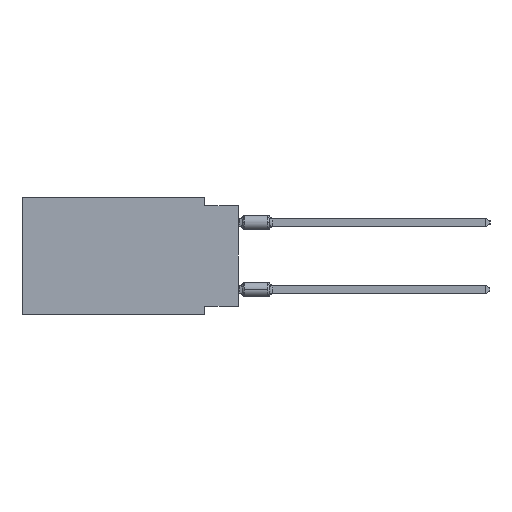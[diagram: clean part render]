
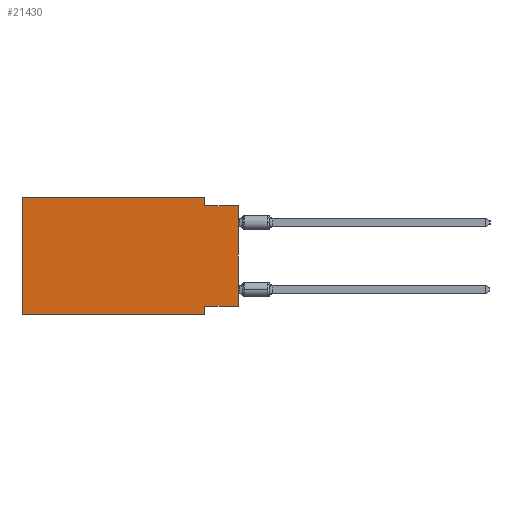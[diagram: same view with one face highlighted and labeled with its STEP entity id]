
A CAD part, left-side view. The second image highlights one B-rep face of the part: STEP entity #21430.
In plain terms, the highlighted planar face has unit normal (-1, 0, 0).
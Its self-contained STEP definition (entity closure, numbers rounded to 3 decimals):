
#437 = PLANE ( 'NONE',  #22385 ) ;
#1089 = LINE ( 'NONE', #18104, #20816 ) ;
#2187 = CARTESIAN_POINT ( 'NONE',  ( 0., 16.383, -8.89 ) ) ;
#2880 = VECTOR ( 'NONE', #39582, 1000. ) ;
#2970 = ORIENTED_EDGE ( 'NONE', *, *, #8130, .T. ) ;
#3034 = EDGE_CURVE ( 'NONE', #49198, #54674, #1089, .T. ) ;
#3231 = VECTOR ( 'NONE', #26576, 1000. ) ;
#4536 = EDGE_CURVE ( 'NONE', #9688, #14217, #16787, .T. ) ;
#5107 = EDGE_CURVE ( 'NONE', #48577, #19049, #5271, .T. ) ;
#5271 = LINE ( 'NONE', #25919, #48688 ) ;
#5369 = ORIENTED_EDGE ( 'NONE', *, *, #5107, .F. ) ;
#6031 = CARTESIAN_POINT ( 'NONE',  ( 0., 0., -0.635 ) ) ;
#6118 = DIRECTION ( 'NONE',  ( 0., 0., 1. ) ) ;
#7225 = CARTESIAN_POINT ( 'NONE',  ( 0., 2.54, -0.635 ) ) ;
#7441 = CARTESIAN_POINT ( 'NONE',  ( 0., 16.383, -8.89 ) ) ;
#8130 = EDGE_CURVE ( 'NONE', #13922, #54674, #41264, .T. ) ;
#9395 = CARTESIAN_POINT ( 'NONE',  ( 0., 2.54, 0. ) ) ;
#9688 = VERTEX_POINT ( 'NONE', #10948 ) ;
#10948 = CARTESIAN_POINT ( 'NONE',  ( 0., 16.383, 0. ) ) ;
#11138 = EDGE_CURVE ( 'NONE', #46643, #49198, #14525, .T. ) ;
#12032 = DIRECTION ( 'NONE',  ( 0., -1., 0. ) ) ;
#13807 = CARTESIAN_POINT ( 'NONE',  ( 0., 2.54, -8.255 ) ) ;
#13908 = EDGE_CURVE ( 'NONE', #13922, #9688, #31509, .T. ) ;
#13922 = VERTEX_POINT ( 'NONE', #2187 ) ;
#14217 = VERTEX_POINT ( 'NONE', #9395 ) ;
#14525 = LINE ( 'NONE', #52854, #3231 ) ;
#16787 = LINE ( 'NONE', #45863, #19187 ) ;
#18097 = ORIENTED_EDGE ( 'NONE', *, *, #24493, .F. ) ;
#18104 = CARTESIAN_POINT ( 'NONE',  ( 0., 2.54, -8.89 ) ) ;
#18314 = LINE ( 'NONE', #35376, #2880 ) ;
#19049 = VERTEX_POINT ( 'NONE', #6031 ) ;
#19088 = VECTOR ( 'NONE', #6118, 1000. ) ;
#19187 = VECTOR ( 'NONE', #12032, 1000. ) ;
#20816 = VECTOR ( 'NONE', #32611, 1000. ) ;
#21430 = ADVANCED_FACE ( 'NONE', ( #38712 ), #437, .F. ) ;
#21928 = CARTESIAN_POINT ( 'NONE',  ( 0., 16.383, 0. ) ) ;
#22385 = AXIS2_PLACEMENT_3D ( 'NONE', #21928, #22477, #51871 ) ;
#22477 = DIRECTION ( 'NONE',  ( 1., 0., 0. ) ) ;
#24463 = DIRECTION ( 'NONE',  ( 0., -1., 0. ) ) ;
#24493 = EDGE_CURVE ( 'NONE', #14217, #48577, #18314, .T. ) ;
#25224 = LINE ( 'NONE', #42289, #30859 ) ;
#25501 = DIRECTION ( 'NONE',  ( 0., 0., 1. ) ) ;
#25919 = CARTESIAN_POINT ( 'NONE',  ( 0., 0., -0.635 ) ) ;
#26576 = DIRECTION ( 'NONE',  ( 0., 1., 0. ) ) ;
#27475 = EDGE_LOOP ( 'NONE', ( #53569, #5369, #18097, #41727, #51964, #2970, #37022, #55034 ) ) ;
#30859 = VECTOR ( 'NONE', #25501, 1000. ) ;
#31509 = LINE ( 'NONE', #49147, #19088 ) ;
#32611 = DIRECTION ( 'NONE',  ( 0., 0., -1. ) ) ;
#32877 = CARTESIAN_POINT ( 'NONE',  ( 0., 0., -8.255 ) ) ;
#35376 = CARTESIAN_POINT ( 'NONE',  ( 0., 2.54, 0. ) ) ;
#37022 = ORIENTED_EDGE ( 'NONE', *, *, #3034, .F. ) ;
#38712 = FACE_OUTER_BOUND ( 'NONE', #27475, .T. ) ;
#39083 = DIRECTION ( 'NONE',  ( 0., -1., 0. ) ) ;
#39582 = DIRECTION ( 'NONE',  ( 0., 0., -1. ) ) ;
#41264 = LINE ( 'NONE', #7441, #53336 ) ;
#41727 = ORIENTED_EDGE ( 'NONE', *, *, #4536, .F. ) ;
#42289 = CARTESIAN_POINT ( 'NONE',  ( 0., 0., 0. ) ) ;
#45863 = CARTESIAN_POINT ( 'NONE',  ( 0., 16.383, 0. ) ) ;
#46358 = CARTESIAN_POINT ( 'NONE',  ( 0., 2.54, -8.89 ) ) ;
#46643 = VERTEX_POINT ( 'NONE', #32877 ) ;
#48577 = VERTEX_POINT ( 'NONE', #7225 ) ;
#48688 = VECTOR ( 'NONE', #39083, 1000. ) ;
#49147 = CARTESIAN_POINT ( 'NONE',  ( 0., 16.383, 0. ) ) ;
#49198 = VERTEX_POINT ( 'NONE', #13807 ) ;
#50789 = EDGE_CURVE ( 'NONE', #46643, #19049, #25224, .T. ) ;
#51871 = DIRECTION ( 'NONE',  ( 0., 0., -1. ) ) ;
#51964 = ORIENTED_EDGE ( 'NONE', *, *, #13908, .F. ) ;
#52854 = CARTESIAN_POINT ( 'NONE',  ( 0., 0., -8.255 ) ) ;
#53336 = VECTOR ( 'NONE', #24463, 1000. ) ;
#53569 = ORIENTED_EDGE ( 'NONE', *, *, #50789, .T. ) ;
#54674 = VERTEX_POINT ( 'NONE', #46358 ) ;
#55034 = ORIENTED_EDGE ( 'NONE', *, *, #11138, .F. ) ;
